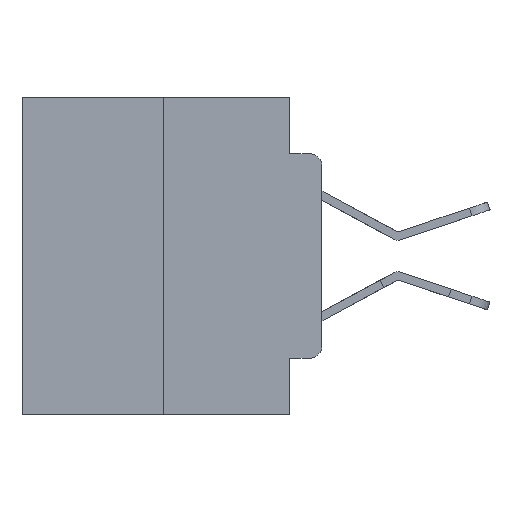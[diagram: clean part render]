
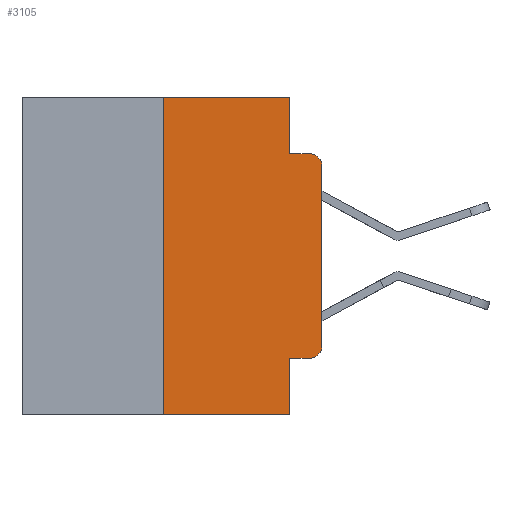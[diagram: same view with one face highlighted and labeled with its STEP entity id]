
A CAD part, left-side view. The second image highlights one B-rep face of the part: STEP entity #3105.
In plain terms, the highlighted planar face has unit normal (-1, 0, 0).
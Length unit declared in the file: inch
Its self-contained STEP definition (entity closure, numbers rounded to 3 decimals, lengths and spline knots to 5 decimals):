
#405 = CARTESIAN_POINT ( 'NONE',  ( 0., 0.051, -0.4115 ) ) ;
#546 = EDGE_CURVE ( 'NONE', #4189, #26894, #14537, .T. ) ;
#1728 = EDGE_CURVE ( 'NONE', #17992, #19404, #14796, .T. ) ;
#1750 = DIRECTION ( 'NONE',  ( -1., 0., 0. ) ) ;
#1937 = EDGE_CURVE ( 'NONE', #12435, #19404, #6479, .T. ) ;
#2369 = CIRCLE ( 'NONE', #21260, 0.02 ) ;
#2856 = VECTOR ( 'NONE', #24798, 39.37008 ) ;
#2930 = DIRECTION ( 'NONE',  ( 0., 0., -1. ) ) ;
#3105 = ADVANCED_FACE ( 'NONE', ( #4427 ), #16528, .F. ) ;
#3655 = CARTESIAN_POINT ( 'NONE',  ( 0., 0.02, -0.4115 ) ) ;
#4128 = CARTESIAN_POINT ( 'NONE',  ( 0., 0., -0.3915 ) ) ;
#4189 = VERTEX_POINT ( 'NONE', #405 ) ;
#4311 = VERTEX_POINT ( 'NONE', #21161 ) ;
#4427 = FACE_OUTER_BOUND ( 'NONE', #16769, .T. ) ;
#4571 = VERTEX_POINT ( 'NONE', #25486 ) ;
#4687 = VECTOR ( 'NONE', #16127, 39.37008 ) ;
#5087 = LINE ( 'NONE', #24439, #9779 ) ;
#5124 = EDGE_CURVE ( 'NONE', #4311, #13737, #20306, .T. ) ;
#5719 = ORIENTED_EDGE ( 'NONE', *, *, #10166, .T. ) ;
#5990 = CARTESIAN_POINT ( 'NONE',  ( 0., 0.051, 0. ) ) ;
#6060 = CARTESIAN_POINT ( 'NONE',  ( 0., 0.02, -0.0885 ) ) ;
#6479 = LINE ( 'NONE', #18425, #2856 ) ;
#6611 = ORIENTED_EDGE ( 'NONE', *, *, #9789, .T. ) ;
#7500 = CARTESIAN_POINT ( 'NONE',  ( 0., 0.051, -0.4115 ) ) ;
#7559 = VECTOR ( 'NONE', #20932, 39.37008 ) ;
#7896 = CARTESIAN_POINT ( 'NONE',  ( 0., 0.051, 0. ) ) ;
#8142 = ORIENTED_EDGE ( 'NONE', *, *, #1937, .F. ) ;
#8376 = ORIENTED_EDGE ( 'NONE', *, *, #13846, .F. ) ;
#9725 = CARTESIAN_POINT ( 'NONE',  ( 0., 0., 0. ) ) ;
#9779 = VECTOR ( 'NONE', #20335, 39.37008 ) ;
#9789 = EDGE_CURVE ( 'NONE', #4571, #26894, #21471, .T. ) ;
#10141 = CARTESIAN_POINT ( 'NONE',  ( 0., 0.473, 0. ) ) ;
#10166 = EDGE_CURVE ( 'NONE', #21925, #17992, #13089, .T. ) ;
#10414 = VECTOR ( 'NONE', #16680, 39.37008 ) ;
#10638 = ORIENTED_EDGE ( 'NONE', *, *, #26304, .F. ) ;
#11120 = LINE ( 'NONE', #16522, #12446 ) ;
#11139 = CARTESIAN_POINT ( 'NONE',  ( 0., 0.473, 0. ) ) ;
#11662 = AXIS2_PLACEMENT_3D ( 'NONE', #10141, #20871, #20960 ) ;
#11859 = EDGE_CURVE ( 'NONE', #22455, #21925, #2369, .T. ) ;
#12116 = AXIS2_PLACEMENT_3D ( 'NONE', #15256, #23975, #2930 ) ;
#12435 = VERTEX_POINT ( 'NONE', #25210 ) ;
#12446 = VECTOR ( 'NONE', #21293, 39.37008 ) ;
#12483 = ORIENTED_EDGE ( 'NONE', *, *, #1728, .T. ) ;
#13089 = LINE ( 'NONE', #9725, #18114 ) ;
#13737 = VERTEX_POINT ( 'NONE', #7896 ) ;
#13846 = EDGE_CURVE ( 'NONE', #13737, #12435, #11120, .T. ) ;
#14537 = LINE ( 'NONE', #5990, #7559 ) ;
#14722 = CARTESIAN_POINT ( 'NONE',  ( 0., 0.473, -0.5 ) ) ;
#14796 = CIRCLE ( 'NONE', #12116, 0.02 ) ;
#15256 = CARTESIAN_POINT ( 'NONE',  ( 0., 0.02, -0.1085 ) ) ;
#16127 = DIRECTION ( 'NONE',  ( 0., -1., 0. ) ) ;
#16319 = LINE ( 'NONE', #7500, #4687 ) ;
#16522 = CARTESIAN_POINT ( 'NONE',  ( 0., 0.051, 0. ) ) ;
#16528 = PLANE ( 'NONE',  #11662 ) ;
#16663 = DIRECTION ( 'NONE',  ( 0., 0., -1. ) ) ;
#16680 = DIRECTION ( 'NONE',  ( 0., -1., 0. ) ) ;
#16769 = EDGE_LOOP ( 'NONE', ( #5719, #12483, #8142, #8376, #25485, #10638, #6611, #22403, #25026, #24923 ) ) ;
#17992 = VERTEX_POINT ( 'NONE', #20343 ) ;
#18114 = VECTOR ( 'NONE', #24835, 39.37008 ) ;
#18425 = CARTESIAN_POINT ( 'NONE',  ( 0., 0.051, -0.0885 ) ) ;
#19404 = VERTEX_POINT ( 'NONE', #6060 ) ;
#20306 = LINE ( 'NONE', #11139, #23959 ) ;
#20335 = DIRECTION ( 'NONE',  ( 0., 0., 1. ) ) ;
#20343 = CARTESIAN_POINT ( 'NONE',  ( 0., 0., -0.1085 ) ) ;
#20871 = DIRECTION ( 'NONE',  ( 1., 0., 0. ) ) ;
#20932 = DIRECTION ( 'NONE',  ( 0., 0., -1. ) ) ;
#20960 = DIRECTION ( 'NONE',  ( 0., 0., -1. ) ) ;
#21158 = CARTESIAN_POINT ( 'NONE',  ( 0., 0.02, -0.3915 ) ) ;
#21161 = CARTESIAN_POINT ( 'NONE',  ( 0., 0.25, 0. ) ) ;
#21260 = AXIS2_PLACEMENT_3D ( 'NONE', #21158, #1750, #16663 ) ;
#21293 = DIRECTION ( 'NONE',  ( 0., 0., -1. ) ) ;
#21471 = LINE ( 'NONE', #14722, #10414 ) ;
#21612 = EDGE_CURVE ( 'NONE', #4189, #22455, #16319, .T. ) ;
#21925 = VERTEX_POINT ( 'NONE', #4128 ) ;
#22403 = ORIENTED_EDGE ( 'NONE', *, *, #546, .F. ) ;
#22455 = VERTEX_POINT ( 'NONE', #3655 ) ;
#23959 = VECTOR ( 'NONE', #26084, 39.37008 ) ;
#23975 = DIRECTION ( 'NONE',  ( -1., 0., 0. ) ) ;
#24439 = CARTESIAN_POINT ( 'NONE',  ( 0., 0.25, 0. ) ) ;
#24509 = CARTESIAN_POINT ( 'NONE',  ( 0., 0.051, -0.5 ) ) ;
#24798 = DIRECTION ( 'NONE',  ( 0., -1., 0. ) ) ;
#24835 = DIRECTION ( 'NONE',  ( 0., 0., 1. ) ) ;
#24923 = ORIENTED_EDGE ( 'NONE', *, *, #11859, .T. ) ;
#25026 = ORIENTED_EDGE ( 'NONE', *, *, #21612, .T. ) ;
#25210 = CARTESIAN_POINT ( 'NONE',  ( 0., 0.051, -0.0885 ) ) ;
#25485 = ORIENTED_EDGE ( 'NONE', *, *, #5124, .F. ) ;
#25486 = CARTESIAN_POINT ( 'NONE',  ( 0., 0.25, -0.5 ) ) ;
#26084 = DIRECTION ( 'NONE',  ( 0., -1., 0. ) ) ;
#26304 = EDGE_CURVE ( 'NONE', #4571, #4311, #5087, .T. ) ;
#26894 = VERTEX_POINT ( 'NONE', #24509 ) ;
